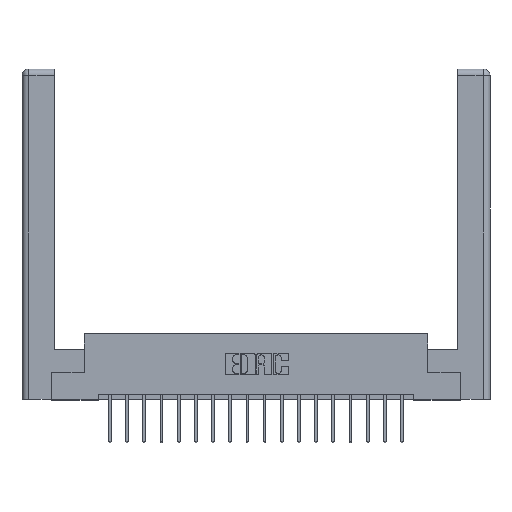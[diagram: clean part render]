
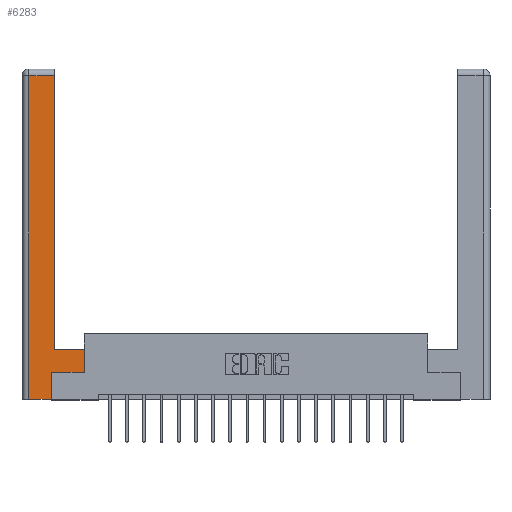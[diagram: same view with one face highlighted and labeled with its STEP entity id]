
A CAD part, top view. The second image highlights one B-rep face of the part: STEP entity #6283.
In plain terms, the highlighted planar face has unit normal (0, 0, 1).
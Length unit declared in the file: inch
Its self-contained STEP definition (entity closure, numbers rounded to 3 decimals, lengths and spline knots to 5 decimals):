
#343 = PLANE ( 'NONE',  #10489 ) ;
#750 = CARTESIAN_POINT ( 'NONE',  ( 0.565, 0.45, 0. ) ) ;
#925 = VECTOR ( 'NONE', #5045, 39.37008 ) ;
#979 = CARTESIAN_POINT ( 'NONE',  ( 0.295, 0.45, 0. ) ) ;
#989 = CARTESIAN_POINT ( 'NONE',  ( 0.295, 0.45, 0. ) ) ;
#1224 = VERTEX_POINT ( 'NONE', #750 ) ;
#1427 = DIRECTION ( 'NONE',  ( 0., 0., -1. ) ) ;
#1771 = VECTOR ( 'NONE', #5496, 39.37008 ) ;
#1881 = ORIENTED_EDGE ( 'NONE', *, *, #15636, .T. ) ;
#1929 = FACE_OUTER_BOUND ( 'NONE', #13286, .T. ) ;
#2383 = DIRECTION ( 'NONE',  ( -1., 0., 0. ) ) ;
#2476 = CARTESIAN_POINT ( 'NONE',  ( 0.265, 0., 0. ) ) ;
#2508 = CARTESIAN_POINT ( 'NONE',  ( 0.265, 0.245, 0. ) ) ;
#2525 = EDGE_CURVE ( 'NONE', #5289, #8727, #2780, .T. ) ;
#2780 = LINE ( 'NONE', #2508, #11841 ) ;
#2873 = ORIENTED_EDGE ( 'NONE', *, *, #8018, .T. ) ;
#3359 = CARTESIAN_POINT ( 'NONE',  ( 0.565, 0.245, 0. ) ) ;
#3613 = DIRECTION ( 'NONE',  ( -1., 0., 0. ) ) ;
#3927 = LINE ( 'NONE', #3965, #1771 ) ;
#3960 = EDGE_CURVE ( 'NONE', #8727, #18711, #13440, .T. ) ;
#3965 = CARTESIAN_POINT ( 'NONE',  ( 0.0615, 0., 0. ) ) ;
#5018 = EDGE_CURVE ( 'NONE', #18711, #1224, #10559, .T. ) ;
#5045 = DIRECTION ( 'NONE',  ( 0., 1., 0. ) ) ;
#5289 = VERTEX_POINT ( 'NONE', #2476 ) ;
#5496 = DIRECTION ( 'NONE',  ( 0., -1., 0. ) ) ;
#5644 = DIRECTION ( 'NONE',  ( -1., 0., 0. ) ) ;
#6283 = ADVANCED_FACE ( 'NONE', ( #1929 ), #343, .F. ) ;
#6528 = CARTESIAN_POINT ( 'NONE',  ( 0.0615, 2.94, 0. ) ) ;
#6952 = VERTEX_POINT ( 'NONE', #17454 ) ;
#7047 = ORIENTED_EDGE ( 'NONE', *, *, #2525, .T. ) ;
#7160 = DIRECTION ( 'NONE',  ( 0., 1., 0. ) ) ;
#7675 = VECTOR ( 'NONE', #12363, 39.37008 ) ;
#8018 = EDGE_CURVE ( 'NONE', #1224, #9236, #9244, .T. ) ;
#8097 = DIRECTION ( 'NONE',  ( 1., 0., 0. ) ) ;
#8187 = ORIENTED_EDGE ( 'NONE', *, *, #11236, .T. ) ;
#8727 = VERTEX_POINT ( 'NONE', #17288 ) ;
#9236 = VERTEX_POINT ( 'NONE', #979 ) ;
#9244 = LINE ( 'NONE', #989, #9960 ) ;
#9532 = CARTESIAN_POINT ( 'NONE',  ( 0., 0., 0. ) ) ;
#9960 = VECTOR ( 'NONE', #2383, 39.37008 ) ;
#10473 = VERTEX_POINT ( 'NONE', #17955 ) ;
#10489 = AXIS2_PLACEMENT_3D ( 'NONE', #9532, #1427, #5644 ) ;
#10559 = LINE ( 'NONE', #10788, #7675 ) ;
#10788 = CARTESIAN_POINT ( 'NONE',  ( 0.565, 0.45, 0. ) ) ;
#10966 = ORIENTED_EDGE ( 'NONE', *, *, #3960, .T. ) ;
#11236 = EDGE_CURVE ( 'NONE', #10473, #14950, #3927, .T. ) ;
#11841 = VECTOR ( 'NONE', #7160, 39.37008 ) ;
#12363 = DIRECTION ( 'NONE',  ( 0., 1., 0. ) ) ;
#12389 = ORIENTED_EDGE ( 'NONE', *, *, #5018, .T. ) ;
#12855 = LINE ( 'NONE', #14161, #925 ) ;
#13286 = EDGE_LOOP ( 'NONE', ( #14391, #17796, #8187, #1881, #7047, #10966, #12389, #2873 ) ) ;
#13440 = LINE ( 'NONE', #14283, #17997 ) ;
#14033 = VECTOR ( 'NONE', #8097, 39.37008 ) ;
#14161 = CARTESIAN_POINT ( 'NONE',  ( 0.295, 3., 0. ) ) ;
#14283 = CARTESIAN_POINT ( 'NONE',  ( 0.565, 0.245, 0. ) ) ;
#14391 = ORIENTED_EDGE ( 'NONE', *, *, #15874, .T. ) ;
#14950 = VERTEX_POINT ( 'NONE', #16184 ) ;
#15636 = EDGE_CURVE ( 'NONE', #14950, #5289, #17634, .T. ) ;
#15874 = EDGE_CURVE ( 'NONE', #9236, #6952, #12855, .T. ) ;
#16184 = CARTESIAN_POINT ( 'NONE',  ( 0.0615, 0., 0. ) ) ;
#17067 = LINE ( 'NONE', #6528, #19679 ) ;
#17288 = CARTESIAN_POINT ( 'NONE',  ( 0.265, 0.245, 0. ) ) ;
#17454 = CARTESIAN_POINT ( 'NONE',  ( 0.295, 2.94, 0. ) ) ;
#17609 = EDGE_CURVE ( 'NONE', #6952, #10473, #17067, .T. ) ;
#17634 = LINE ( 'NONE', #18872, #14033 ) ;
#17796 = ORIENTED_EDGE ( 'NONE', *, *, #17609, .T. ) ;
#17955 = CARTESIAN_POINT ( 'NONE',  ( 0.0615, 2.94, 0. ) ) ;
#17997 = VECTOR ( 'NONE', #18956, 39.37008 ) ;
#18711 = VERTEX_POINT ( 'NONE', #3359 ) ;
#18872 = CARTESIAN_POINT ( 'NONE',  ( 0.265, 0., 0. ) ) ;
#18956 = DIRECTION ( 'NONE',  ( 1., 0., 0. ) ) ;
#19679 = VECTOR ( 'NONE', #3613, 39.37008 ) ;
